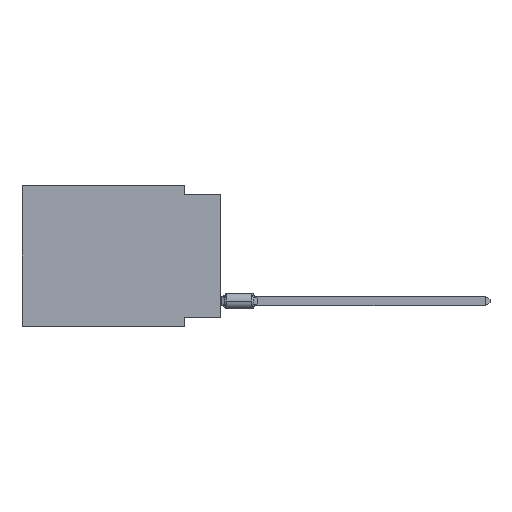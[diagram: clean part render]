
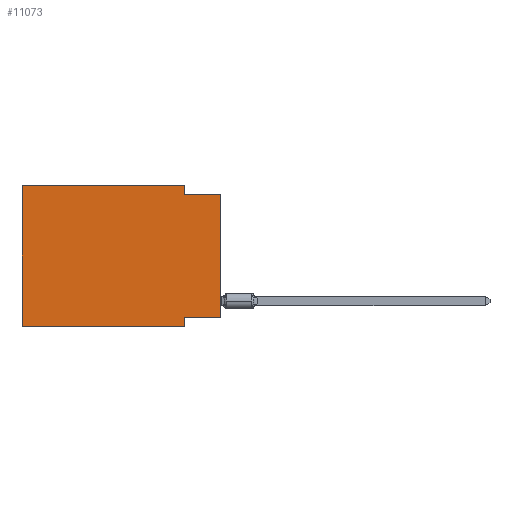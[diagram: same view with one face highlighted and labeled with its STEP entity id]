
A CAD part, left-side view. The second image highlights one B-rep face of the part: STEP entity #11073.
In plain terms, the highlighted planar face has unit normal (-1, 0, 0).
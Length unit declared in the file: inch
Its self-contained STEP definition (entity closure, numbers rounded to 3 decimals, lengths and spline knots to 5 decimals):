
#323 = EDGE_CURVE ( 'NONE', #73367, #64453, #53286, .T. ) ;
#730 = EDGE_CURVE ( 'NONE', #1762, #19417, #46925, .T. ) ;
#1762 = VERTEX_POINT ( 'NONE', #42764 ) ;
#2368 = ORIENTED_EDGE ( 'NONE', *, *, #47988, .F. ) ;
#4401 = CARTESIAN_POINT ( 'NONE',  ( 0., 0., -0.365 ) ) ;
#4651 = LINE ( 'NONE', #75301, #42095 ) ;
#5551 = DIRECTION ( 'NONE',  ( 0., -1., 0. ) ) ;
#6179 = VECTOR ( 'NONE', #5551, 39.37008 ) ;
#11073 = ADVANCED_FACE ( 'NONE', ( #76646 ), #35260, .F. ) ;
#11844 = CARTESIAN_POINT ( 'NONE',  ( 0., 0.55, 0. ) ) ;
#11930 = VECTOR ( 'NONE', #16481, 39.37008 ) ;
#16481 = DIRECTION ( 'NONE',  ( 0., 1., 0. ) ) ;
#17636 = CARTESIAN_POINT ( 'NONE',  ( 0., 0.55, -0.39 ) ) ;
#19417 = VERTEX_POINT ( 'NONE', #25950 ) ;
#19547 = AXIS2_PLACEMENT_3D ( 'NONE', #11844, #30191, #71176 ) ;
#20555 = LINE ( 'NONE', #61920, #47653 ) ;
#24038 = EDGE_CURVE ( 'NONE', #52541, #24875, #4651, .T. ) ;
#24875 = VERTEX_POINT ( 'NONE', #63302 ) ;
#25950 = CARTESIAN_POINT ( 'NONE',  ( 0., 0.1, -0.365 ) ) ;
#26770 = CARTESIAN_POINT ( 'NONE',  ( 0., 0., -0.025 ) ) ;
#28816 = EDGE_CURVE ( 'NONE', #1762, #35529, #60150, .T. ) ;
#30191 = DIRECTION ( 'NONE',  ( 1., 0., 0. ) ) ;
#31454 = ORIENTED_EDGE ( 'NONE', *, *, #730, .F. ) ;
#31475 = EDGE_CURVE ( 'NONE', #24875, #73367, #20555, .T. ) ;
#32256 = VECTOR ( 'NONE', #47421, 39.37008 ) ;
#32707 = CARTESIAN_POINT ( 'NONE',  ( 0., 0.1, -0.39 ) ) ;
#34696 = ORIENTED_EDGE ( 'NONE', *, *, #37477, .T. ) ;
#35260 = PLANE ( 'NONE',  #19547 ) ;
#35261 = VECTOR ( 'NONE', #47750, 39.37008 ) ;
#35529 = VERTEX_POINT ( 'NONE', #45026 ) ;
#36546 = VERTEX_POINT ( 'NONE', #32707 ) ;
#37477 = EDGE_CURVE ( 'NONE', #52541, #36546, #58235, .T. ) ;
#39876 = VECTOR ( 'NONE', #65994, 39.37008 ) ;
#42095 = VECTOR ( 'NONE', #45259, 39.37008 ) ;
#42764 = CARTESIAN_POINT ( 'NONE',  ( 0., 0., -0.365 ) ) ;
#44286 = ORIENTED_EDGE ( 'NONE', *, *, #72212, .F. ) ;
#45026 = CARTESIAN_POINT ( 'NONE',  ( 0., 0., -0.025 ) ) ;
#45259 = DIRECTION ( 'NONE',  ( 0., 0., 1. ) ) ;
#45278 = VECTOR ( 'NONE', #50588, 39.37008 ) ;
#46925 = LINE ( 'NONE', #4401, #11930 ) ;
#47421 = DIRECTION ( 'NONE',  ( 0., 0., -1. ) ) ;
#47653 = VECTOR ( 'NONE', #66626, 39.37008 ) ;
#47750 = DIRECTION ( 'NONE',  ( 0., 0., -1. ) ) ;
#47988 = EDGE_CURVE ( 'NONE', #64453, #35529, #54921, .T. ) ;
#50588 = DIRECTION ( 'NONE',  ( 0., -1., 0. ) ) ;
#51204 = ORIENTED_EDGE ( 'NONE', *, *, #24038, .F. ) ;
#52541 = VERTEX_POINT ( 'NONE', #64380 ) ;
#53286 = LINE ( 'NONE', #58737, #32256 ) ;
#54694 = CARTESIAN_POINT ( 'NONE',  ( 0., 0., 0. ) ) ;
#54921 = LINE ( 'NONE', #26770, #45278 ) ;
#56329 = CARTESIAN_POINT ( 'NONE',  ( 0., 0.1, -0.025 ) ) ;
#58235 = LINE ( 'NONE', #17636, #6179 ) ;
#58255 = ORIENTED_EDGE ( 'NONE', *, *, #31475, .F. ) ;
#58737 = CARTESIAN_POINT ( 'NONE',  ( 0., 0.1, 0. ) ) ;
#60150 = LINE ( 'NONE', #54694, #39876 ) ;
#60373 = ORIENTED_EDGE ( 'NONE', *, *, #28816, .T. ) ;
#60557 = CARTESIAN_POINT ( 'NONE',  ( 0., 0.1, 0. ) ) ;
#61920 = CARTESIAN_POINT ( 'NONE',  ( 0., 0.55, 0. ) ) ;
#63302 = CARTESIAN_POINT ( 'NONE',  ( 0., 0.55, 0. ) ) ;
#64380 = CARTESIAN_POINT ( 'NONE',  ( 0., 0.55, -0.39 ) ) ;
#64453 = VERTEX_POINT ( 'NONE', #56329 ) ;
#65676 = LINE ( 'NONE', #71552, #35261 ) ;
#65994 = DIRECTION ( 'NONE',  ( 0., 0., 1. ) ) ;
#66509 = ORIENTED_EDGE ( 'NONE', *, *, #323, .F. ) ;
#66626 = DIRECTION ( 'NONE',  ( 0., -1., 0. ) ) ;
#70181 = EDGE_LOOP ( 'NONE', ( #60373, #2368, #66509, #58255, #51204, #34696, #44286, #31454 ) ) ;
#71176 = DIRECTION ( 'NONE',  ( 0., 0., -1. ) ) ;
#71552 = CARTESIAN_POINT ( 'NONE',  ( 0., 0.1, -0.39 ) ) ;
#72212 = EDGE_CURVE ( 'NONE', #19417, #36546, #65676, .T. ) ;
#73367 = VERTEX_POINT ( 'NONE', #60557 ) ;
#75301 = CARTESIAN_POINT ( 'NONE',  ( 0., 0.55, 0. ) ) ;
#76646 = FACE_OUTER_BOUND ( 'NONE', #70181, .T. ) ;
